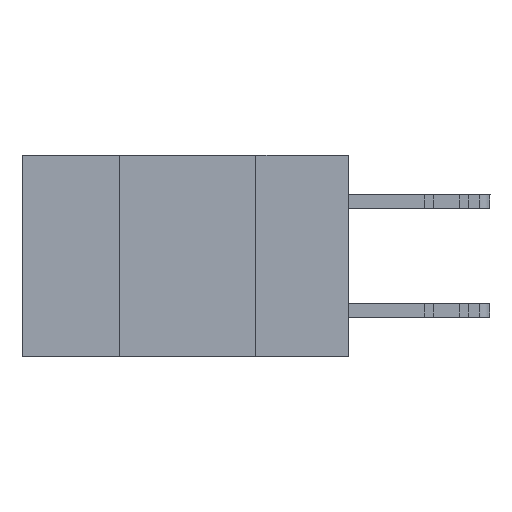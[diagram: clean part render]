
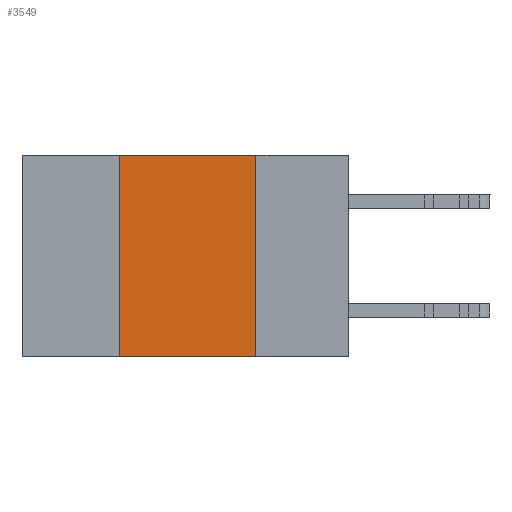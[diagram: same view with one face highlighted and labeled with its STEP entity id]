
A CAD part, left-side view. The second image highlights one B-rep face of the part: STEP entity #3549.
In plain terms, the highlighted planar face has unit normal (-1, 0, 0).
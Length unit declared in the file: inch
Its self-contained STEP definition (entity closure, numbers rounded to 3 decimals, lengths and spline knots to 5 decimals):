
#117 = EDGE_CURVE ( 'NONE', #27156, #20755, #21991, .T. ) ;
#169 = VERTEX_POINT ( 'NONE', #14217 ) ;
#503 = EDGE_LOOP ( 'NONE', ( #6327, #21203, #32898, #27120 ) ) ;
#2274 = CARTESIAN_POINT ( 'NONE',  ( 0., 0.42, 0. ) ) ;
#2385 = DIRECTION ( 'NONE',  ( 0., -1., 0. ) ) ;
#2514 = VECTOR ( 'NONE', #2385, 39.37008 ) ;
#2607 = LINE ( 'NONE', #2274, #28212 ) ;
#3549 = ADVANCED_FACE ( 'NONE', ( #7877 ), #28109, .F. ) ;
#3810 = CARTESIAN_POINT ( 'NONE',  ( 0., 0.17, 0. ) ) ;
#4994 = DIRECTION ( 'NONE',  ( 0., 0., 1. ) ) ;
#5473 = VECTOR ( 'NONE', #16722, 39.37008 ) ;
#6327 = ORIENTED_EDGE ( 'NONE', *, *, #23928, .F. ) ;
#6348 = EDGE_CURVE ( 'NONE', #27156, #169, #2607, .T. ) ;
#6987 = CARTESIAN_POINT ( 'NONE',  ( 0., 0.42, -0.37 ) ) ;
#7877 = FACE_OUTER_BOUND ( 'NONE', #503, .T. ) ;
#10909 = VERTEX_POINT ( 'NONE', #24230 ) ;
#11106 = DIRECTION ( 'NONE',  ( 0., 0., -1. ) ) ;
#14217 = CARTESIAN_POINT ( 'NONE',  ( 0., 0.42, 0. ) ) ;
#15979 = LINE ( 'NONE', #3810, #20341 ) ;
#16597 = CARTESIAN_POINT ( 'NONE',  ( 0., 0.17, -0.37 ) ) ;
#16722 = DIRECTION ( 'NONE',  ( 0., -1., 0. ) ) ;
#20341 = VECTOR ( 'NONE', #11106, 39.37008 ) ;
#20533 = DIRECTION ( 'NONE',  ( 0., 0., -1. ) ) ;
#20755 = VERTEX_POINT ( 'NONE', #16597 ) ;
#21203 = ORIENTED_EDGE ( 'NONE', *, *, #30268, .F. ) ;
#21484 = CARTESIAN_POINT ( 'NONE',  ( 0., 0.6, -0.37 ) ) ;
#21991 = LINE ( 'NONE', #21484, #5473 ) ;
#22953 = DIRECTION ( 'NONE',  ( 1., 0., 0. ) ) ;
#23166 = AXIS2_PLACEMENT_3D ( 'NONE', #25612, #22953, #20533 ) ;
#23928 = EDGE_CURVE ( 'NONE', #10909, #20755, #15979, .T. ) ;
#24230 = CARTESIAN_POINT ( 'NONE',  ( 0., 0.17, 0. ) ) ;
#25612 = CARTESIAN_POINT ( 'NONE',  ( 0., 0.6, 0. ) ) ;
#27120 = ORIENTED_EDGE ( 'NONE', *, *, #117, .T. ) ;
#27156 = VERTEX_POINT ( 'NONE', #6987 ) ;
#28109 = PLANE ( 'NONE',  #23166 ) ;
#28212 = VECTOR ( 'NONE', #4994, 39.37008 ) ;
#30268 = EDGE_CURVE ( 'NONE', #169, #10909, #31037, .T. ) ;
#30554 = CARTESIAN_POINT ( 'NONE',  ( 0., 0.6, 0. ) ) ;
#31037 = LINE ( 'NONE', #30554, #2514 ) ;
#32898 = ORIENTED_EDGE ( 'NONE', *, *, #6348, .F. ) ;
